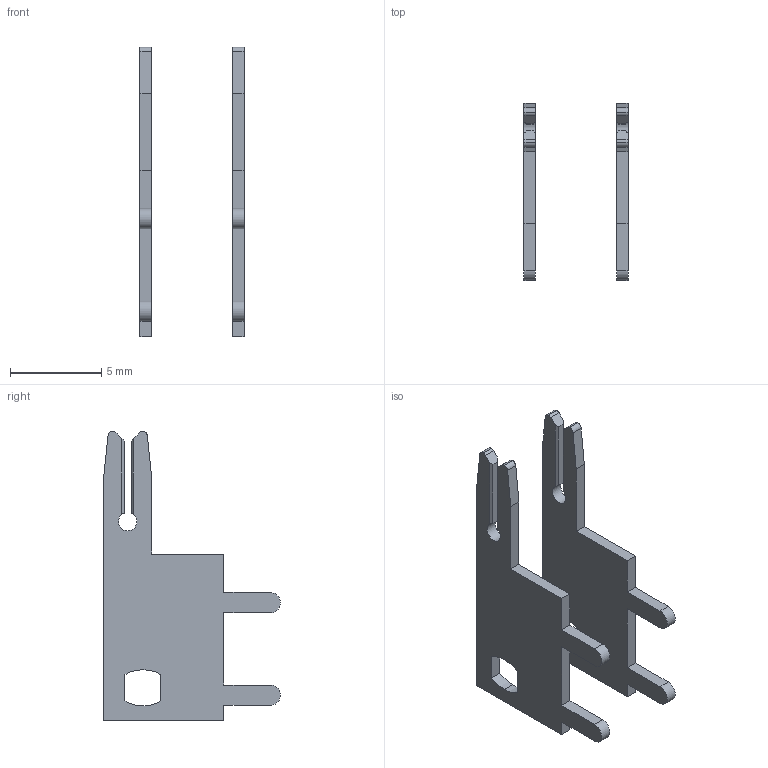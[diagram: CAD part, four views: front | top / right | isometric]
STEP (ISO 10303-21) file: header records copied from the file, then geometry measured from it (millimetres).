
FILE_DESCRIPTION (( 'STEP AP203' ), '1' );
FILE_NAME ('105-002-201-200.STEP', '2020-04-07T22:02:48', ( '' ), ( '' ), 'SwSTEP 2.0', 'SolidWorks 2016', '' );
FILE_SCHEMA (( 'CONFIG_CONTROL_DESIGN' ));
Length unit declared in the file: inch
Products named in the file (2): 100-290-001_100-290-201; 105-002-201-200
Assembly tree (2 placements, depth 2):
  105-002-201-200
    100-290-001_100-290-201  x2
Bounding box: 5.71 x 9.7 x 15.88 mm (x, y, z)
Volume: 98.5 mm3; surface area: 401.9 mm2
Topology: 2 solids, 2 shells, 70 faces, 198 edges, 132 vertices
Faces by surface type: plane 50, cylinder 20
Entity records: 1369 total; most frequent: CARTESIAN_POINT 217, ORIENTED_EDGE 198, DIRECTION 195, EDGE_CURVE 99, LINE 75, VECTOR 75, VERTEX_POINT 66, AXIS2_PLACEMENT_3D 60
